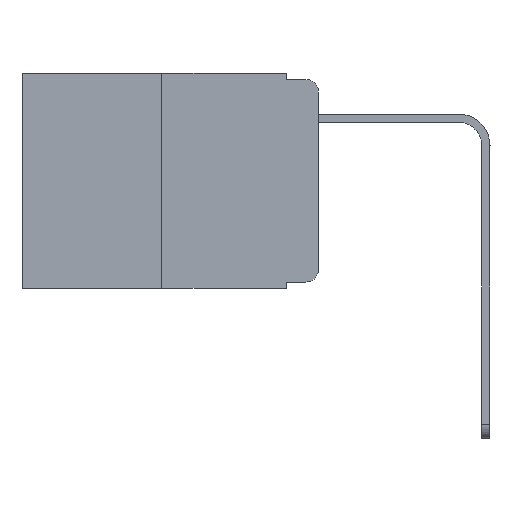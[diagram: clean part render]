
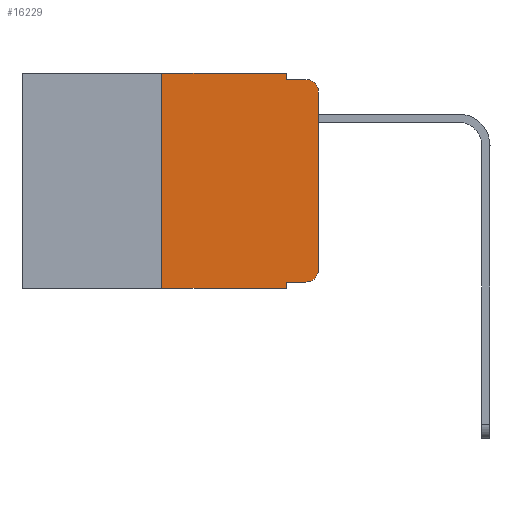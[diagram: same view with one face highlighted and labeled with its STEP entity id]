
A CAD part, left-side view. The second image highlights one B-rep face of the part: STEP entity #16229.
In plain terms, the highlighted planar face has unit normal (-1, 0, 0).
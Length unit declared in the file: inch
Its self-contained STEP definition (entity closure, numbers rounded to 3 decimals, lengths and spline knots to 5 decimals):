
#427 = EDGE_CURVE ( 'NONE', #19552, #7999, #11508, .T. ) ;
#712 = CARTESIAN_POINT ( 'NONE',  ( 0., 0.051, 0. ) ) ;
#925 = DIRECTION ( 'NONE',  ( 0., 0., 1. ) ) ;
#1149 = PLANE ( 'NONE',  #8776 ) ;
#1468 = VERTEX_POINT ( 'NONE', #2623 ) ;
#1626 = CARTESIAN_POINT ( 'NONE',  ( 0., 0.02, -0.03 ) ) ;
#1885 = ORIENTED_EDGE ( 'NONE', *, *, #12172, .F. ) ;
#2145 = CARTESIAN_POINT ( 'NONE',  ( 0., 0.25, -0.343 ) ) ;
#2242 = VECTOR ( 'NONE', #15872, 39.37008 ) ;
#2406 = LINE ( 'NONE', #712, #19513 ) ;
#2623 = CARTESIAN_POINT ( 'NONE',  ( 0., 0., -0.03 ) ) ;
#2872 = DIRECTION ( 'NONE',  ( -1., 0., 0. ) ) ;
#3198 = CARTESIAN_POINT ( 'NONE',  ( 0., 0.25, 0. ) ) ;
#3211 = EDGE_CURVE ( 'NONE', #3475, #13958, #20228, .T. ) ;
#3255 = LINE ( 'NONE', #11157, #2242 ) ;
#3475 = VERTEX_POINT ( 'NONE', #17533 ) ;
#3886 = CARTESIAN_POINT ( 'NONE',  ( 0., 0.473, 0. ) ) ;
#3924 = EDGE_CURVE ( 'NONE', #6904, #11215, #15588, .T. ) ;
#4156 = VECTOR ( 'NONE', #5363, 39.37008 ) ;
#5363 = DIRECTION ( 'NONE',  ( 0., 0., 1. ) ) ;
#5394 = ORIENTED_EDGE ( 'NONE', *, *, #14848, .F. ) ;
#5482 = CARTESIAN_POINT ( 'NONE',  ( 0., 0.051, 0. ) ) ;
#5916 = LINE ( 'NONE', #3198, #4156 ) ;
#6012 = CIRCLE ( 'NONE', #13739, 0.02 ) ;
#6067 = CARTESIAN_POINT ( 'NONE',  ( 0., 0.473, 0. ) ) ;
#6201 = DIRECTION ( 'NONE',  ( 0., 0., -1. ) ) ;
#6364 = VERTEX_POINT ( 'NONE', #8873 ) ;
#6417 = LINE ( 'NONE', #10272, #16897 ) ;
#6904 = VERTEX_POINT ( 'NONE', #14015 ) ;
#7161 = FACE_OUTER_BOUND ( 'NONE', #16012, .T. ) ;
#7999 = VERTEX_POINT ( 'NONE', #19845 ) ;
#8776 = AXIS2_PLACEMENT_3D ( 'NONE', #6067, #17506, #12442 ) ;
#8873 = CARTESIAN_POINT ( 'NONE',  ( 0., 0.051, -0.333 ) ) ;
#9111 = CARTESIAN_POINT ( 'NONE',  ( 0., 0., -0.313 ) ) ;
#9620 = CIRCLE ( 'NONE', #16466, 0.02 ) ;
#9668 = DIRECTION ( 'NONE',  ( -1., 0., 0. ) ) ;
#10096 = VECTOR ( 'NONE', #12012, 39.37008 ) ;
#10272 = CARTESIAN_POINT ( 'NONE',  ( 0., 0., 0. ) ) ;
#10767 = ORIENTED_EDGE ( 'NONE', *, *, #19119, .F. ) ;
#11064 = CARTESIAN_POINT ( 'NONE',  ( 0., 0.02, -0.313 ) ) ;
#11157 = CARTESIAN_POINT ( 'NONE',  ( 0., 0.051, -0.333 ) ) ;
#11215 = VERTEX_POINT ( 'NONE', #19991 ) ;
#11508 = LINE ( 'NONE', #14442, #19169 ) ;
#11788 = VECTOR ( 'NONE', #16976, 39.37008 ) ;
#12012 = DIRECTION ( 'NONE',  ( 0., 0., -1. ) ) ;
#12120 = ORIENTED_EDGE ( 'NONE', *, *, #3924, .F. ) ;
#12164 = DIRECTION ( 'NONE',  ( 0., -1., 0. ) ) ;
#12172 = EDGE_CURVE ( 'NONE', #19552, #6904, #5916, .T. ) ;
#12442 = DIRECTION ( 'NONE',  ( 0., 0., -1. ) ) ;
#12666 = LINE ( 'NONE', #5482, #10096 ) ;
#12718 = ORIENTED_EDGE ( 'NONE', *, *, #12963, .T. ) ;
#12746 = VERTEX_POINT ( 'NONE', #17937 ) ;
#12963 = EDGE_CURVE ( 'NONE', #16230, #1468, #6417, .T. ) ;
#13739 = AXIS2_PLACEMENT_3D ( 'NONE', #11064, #2872, #6201 ) ;
#13958 = VERTEX_POINT ( 'NONE', #19671 ) ;
#14015 = CARTESIAN_POINT ( 'NONE',  ( 0., 0.25, 0. ) ) ;
#14027 = ORIENTED_EDGE ( 'NONE', *, *, #3211, .F. ) ;
#14442 = CARTESIAN_POINT ( 'NONE',  ( 0., 0.473, -0.343 ) ) ;
#14579 = VECTOR ( 'NONE', #12164, 39.37008 ) ;
#14848 = EDGE_CURVE ( 'NONE', #6364, #7999, #2406, .T. ) ;
#15340 = DIRECTION ( 'NONE',  ( 0., 0., -1. ) ) ;
#15551 = ORIENTED_EDGE ( 'NONE', *, *, #19378, .T. ) ;
#15588 = LINE ( 'NONE', #3886, #14579 ) ;
#15872 = DIRECTION ( 'NONE',  ( 0., -1., 0. ) ) ;
#16012 = EDGE_LOOP ( 'NONE', ( #12718, #19134, #14027, #10767, #12120, #1885, #21164, #5394, #19731, #15551 ) ) ;
#16185 = DIRECTION ( 'NONE',  ( 0., 0., -1. ) ) ;
#16229 = ADVANCED_FACE ( 'NONE', ( #7161 ), #1149, .F. ) ;
#16230 = VERTEX_POINT ( 'NONE', #9111 ) ;
#16466 = AXIS2_PLACEMENT_3D ( 'NONE', #1626, #9668, #16185 ) ;
#16897 = VECTOR ( 'NONE', #925, 39.37008 ) ;
#16976 = DIRECTION ( 'NONE',  ( 0., -1., 0. ) ) ;
#17506 = DIRECTION ( 'NONE',  ( 1., 0., 0. ) ) ;
#17533 = CARTESIAN_POINT ( 'NONE',  ( 0., 0.051, -0.01 ) ) ;
#17731 = DIRECTION ( 'NONE',  ( 0., -1., 0. ) ) ;
#17840 = CARTESIAN_POINT ( 'NONE',  ( 0., 0.051, -0.01 ) ) ;
#17937 = CARTESIAN_POINT ( 'NONE',  ( 0., 0.02, -0.333 ) ) ;
#18111 = EDGE_CURVE ( 'NONE', #1468, #13958, #9620, .T. ) ;
#18584 = EDGE_CURVE ( 'NONE', #6364, #12746, #3255, .T. ) ;
#19119 = EDGE_CURVE ( 'NONE', #11215, #3475, #12666, .T. ) ;
#19134 = ORIENTED_EDGE ( 'NONE', *, *, #18111, .T. ) ;
#19169 = VECTOR ( 'NONE', #17731, 39.37008 ) ;
#19378 = EDGE_CURVE ( 'NONE', #12746, #16230, #6012, .T. ) ;
#19513 = VECTOR ( 'NONE', #15340, 39.37008 ) ;
#19552 = VERTEX_POINT ( 'NONE', #2145 ) ;
#19671 = CARTESIAN_POINT ( 'NONE',  ( 0., 0.02, -0.01 ) ) ;
#19731 = ORIENTED_EDGE ( 'NONE', *, *, #18584, .T. ) ;
#19845 = CARTESIAN_POINT ( 'NONE',  ( 0., 0.051, -0.343 ) ) ;
#19991 = CARTESIAN_POINT ( 'NONE',  ( 0., 0.051, 0. ) ) ;
#20228 = LINE ( 'NONE', #17840, #11788 ) ;
#21164 = ORIENTED_EDGE ( 'NONE', *, *, #427, .T. ) ;
